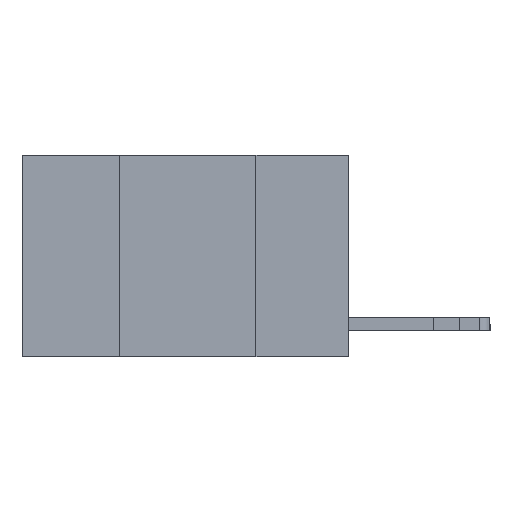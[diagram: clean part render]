
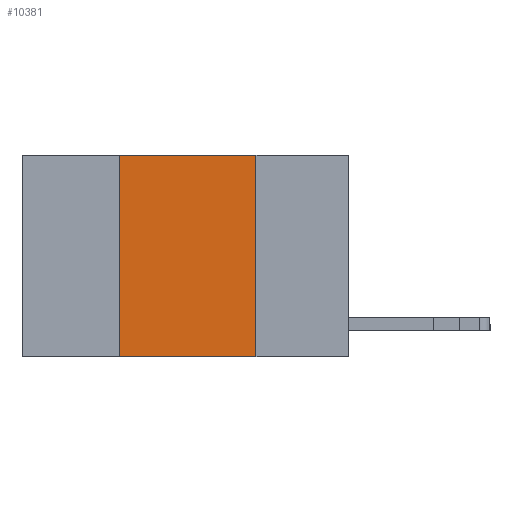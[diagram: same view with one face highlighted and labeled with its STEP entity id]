
A CAD part, left-side view. The second image highlights one B-rep face of the part: STEP entity #10381.
In plain terms, the highlighted planar face has unit normal (-1, 0, 0).
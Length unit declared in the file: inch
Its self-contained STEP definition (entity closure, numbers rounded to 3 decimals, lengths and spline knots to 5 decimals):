
#176 = EDGE_CURVE ( 'NONE', #5687, #11734, #1870, .T. ) ;
#371 = LINE ( 'NONE', #8528, #10995 ) ;
#853 = FACE_OUTER_BOUND ( 'NONE', #10852, .T. ) ;
#1057 = CARTESIAN_POINT ( 'NONE',  ( 0., 0.42, 0. ) ) ;
#1058 = VERTEX_POINT ( 'NONE', #11886 ) ;
#1354 = LINE ( 'NONE', #7394, #3369 ) ;
#1870 = LINE ( 'NONE', #12120, #3032 ) ;
#1974 = VERTEX_POINT ( 'NONE', #1057 ) ;
#2735 = EDGE_CURVE ( 'NONE', #1974, #1058, #10862, .T. ) ;
#2987 = CARTESIAN_POINT ( 'NONE',  ( 0., 0.6, 0. ) ) ;
#3007 = CARTESIAN_POINT ( 'NONE',  ( 0., 0.17, -0.37 ) ) ;
#3024 = EDGE_CURVE ( 'NONE', #5687, #1974, #1354, .T. ) ;
#3032 = VECTOR ( 'NONE', #11917, 39.37008 ) ;
#3369 = VECTOR ( 'NONE', #9657, 39.37008 ) ;
#5687 = VERTEX_POINT ( 'NONE', #8992 ) ;
#7307 = ORIENTED_EDGE ( 'NONE', *, *, #176, .T. ) ;
#7394 = CARTESIAN_POINT ( 'NONE',  ( 0., 0.42, 0. ) ) ;
#8231 = PLANE ( 'NONE',  #9272 ) ;
#8346 = ORIENTED_EDGE ( 'NONE', *, *, #12139, .F. ) ;
#8528 = CARTESIAN_POINT ( 'NONE',  ( 0., 0.17, 0. ) ) ;
#8992 = CARTESIAN_POINT ( 'NONE',  ( 0., 0.42, -0.37 ) ) ;
#9272 = AXIS2_PLACEMENT_3D ( 'NONE', #2987, #12229, #10172 ) ;
#9531 = ORIENTED_EDGE ( 'NONE', *, *, #3024, .F. ) ;
#9657 = DIRECTION ( 'NONE',  ( 0., 0., 1. ) ) ;
#10011 = DIRECTION ( 'NONE',  ( 0., -1., 0. ) ) ;
#10069 = CARTESIAN_POINT ( 'NONE',  ( 0., 0.6, 0. ) ) ;
#10172 = DIRECTION ( 'NONE',  ( 0., 0., -1. ) ) ;
#10381 = ADVANCED_FACE ( 'NONE', ( #853 ), #8231, .F. ) ;
#10541 = DIRECTION ( 'NONE',  ( 0., 0., -1. ) ) ;
#10852 = EDGE_LOOP ( 'NONE', ( #8346, #11068, #9531, #7307 ) ) ;
#10862 = LINE ( 'NONE', #10069, #12939 ) ;
#10995 = VECTOR ( 'NONE', #10541, 39.37008 ) ;
#11068 = ORIENTED_EDGE ( 'NONE', *, *, #2735, .F. ) ;
#11734 = VERTEX_POINT ( 'NONE', #3007 ) ;
#11886 = CARTESIAN_POINT ( 'NONE',  ( 0., 0.17, 0. ) ) ;
#11917 = DIRECTION ( 'NONE',  ( 0., -1., 0. ) ) ;
#12120 = CARTESIAN_POINT ( 'NONE',  ( 0., 0.6, -0.37 ) ) ;
#12139 = EDGE_CURVE ( 'NONE', #1058, #11734, #371, .T. ) ;
#12229 = DIRECTION ( 'NONE',  ( 1., 0., 0. ) ) ;
#12939 = VECTOR ( 'NONE', #10011, 39.37008 ) ;
